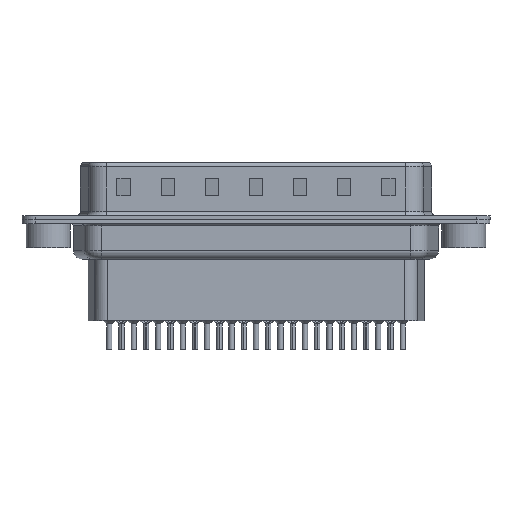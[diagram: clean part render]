
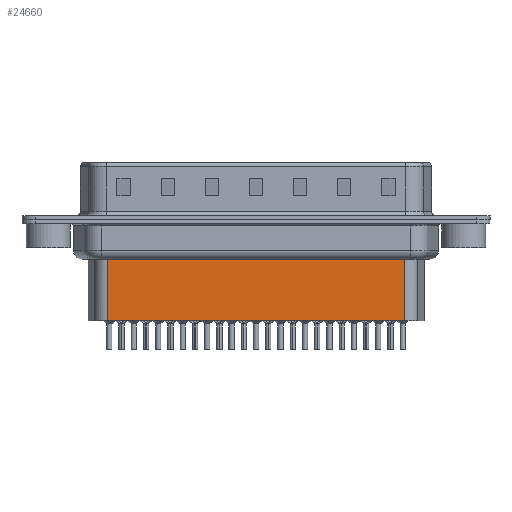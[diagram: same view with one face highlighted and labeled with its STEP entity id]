
A CAD part, front view. The second image highlights one B-rep face of the part: STEP entity #24660.
In plain terms, the highlighted planar face has unit normal (0, -1, 0).
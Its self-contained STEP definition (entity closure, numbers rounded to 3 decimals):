
#425 = CARTESIAN_POINT ( 'NONE',  ( 40.344, -3.5, -11.45 ) ) ;
#542 = DIRECTION ( 'NONE',  ( 0., 0., -1. ) ) ;
#623 = CARTESIAN_POINT ( 'NONE',  ( 6.706, -3.5, -3.1 ) ) ;
#1274 = LINE ( 'NONE', #12115, #21311 ) ;
#2563 = VERTEX_POINT ( 'NONE', #19731 ) ;
#3186 = CARTESIAN_POINT ( 'NONE',  ( 40.344, -3.5, -4.097 ) ) ;
#3290 = EDGE_LOOP ( 'NONE', ( #22523, #12220, #8310, #14249 ) ) ;
#4573 = VECTOR ( 'NONE', #16338, 1000. ) ;
#4821 = LINE ( 'NONE', #13828, #19768 ) ;
#5149 = EDGE_CURVE ( 'NONE', #16621, #2563, #7064, .T. ) ;
#5191 = EDGE_CURVE ( 'NONE', #7712, #16621, #1274, .T. ) ;
#5274 = EDGE_CURVE ( 'NONE', #25037, #2563, #15079, .T. ) ;
#7064 = LINE ( 'NONE', #12779, #21917 ) ;
#7402 = EDGE_CURVE ( 'NONE', #7712, #25037, #4821, .T. ) ;
#7712 = VERTEX_POINT ( 'NONE', #3186 ) ;
#8310 = ORIENTED_EDGE ( 'NONE', *, *, #5274, .T. ) ;
#9171 = DIRECTION ( 'NONE',  ( -1., 0., 0. ) ) ;
#10991 = CARTESIAN_POINT ( 'NONE',  ( 6.706, -3.5, -3.1 ) ) ;
#12115 = CARTESIAN_POINT ( 'NONE',  ( 40.344, -3.5, -3.1 ) ) ;
#12220 = ORIENTED_EDGE ( 'NONE', *, *, #7402, .T. ) ;
#12779 = CARTESIAN_POINT ( 'NONE',  ( 6.706, -3.5, -11.45 ) ) ;
#13003 = DIRECTION ( 'NONE',  ( 1., 0., 0. ) ) ;
#13828 = CARTESIAN_POINT ( 'NONE',  ( 6.459, -3.5, -4.097 ) ) ;
#14238 = CARTESIAN_POINT ( 'NONE',  ( 6.706, -3.5, -4.097 ) ) ;
#14249 = ORIENTED_EDGE ( 'NONE', *, *, #5149, .F. ) ;
#15079 = LINE ( 'NONE', #623, #4573 ) ;
#15704 = FACE_OUTER_BOUND ( 'NONE', #3290, .T. ) ;
#16338 = DIRECTION ( 'NONE',  ( 0., 0., -1. ) ) ;
#16621 = VERTEX_POINT ( 'NONE', #425 ) ;
#19145 = AXIS2_PLACEMENT_3D ( 'NONE', #10991, #24545, #13003 ) ;
#19731 = CARTESIAN_POINT ( 'NONE',  ( 6.706, -3.5, -11.45 ) ) ;
#19768 = VECTOR ( 'NONE', #21388, 1000. ) ;
#21311 = VECTOR ( 'NONE', #542, 1000. ) ;
#21388 = DIRECTION ( 'NONE',  ( -1., 0., 0. ) ) ;
#21917 = VECTOR ( 'NONE', #9171, 1000. ) ;
#22523 = ORIENTED_EDGE ( 'NONE', *, *, #5191, .F. ) ;
#22541 = PLANE ( 'NONE',  #19145 ) ;
#24545 = DIRECTION ( 'NONE',  ( 0., -1., 0. ) ) ;
#24660 = ADVANCED_FACE ( 'NONE', ( #15704 ), #22541, .T. ) ;
#25037 = VERTEX_POINT ( 'NONE', #14238 ) ;
